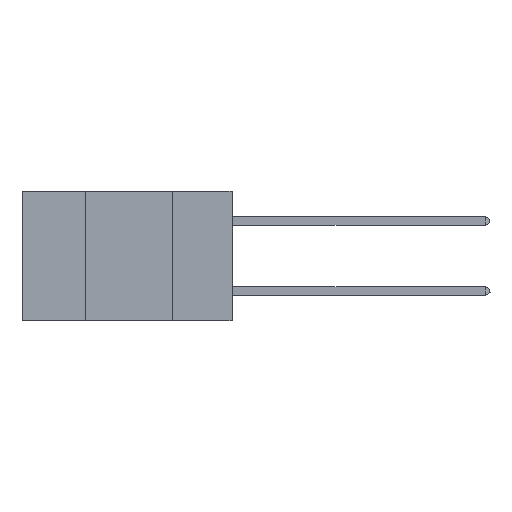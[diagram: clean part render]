
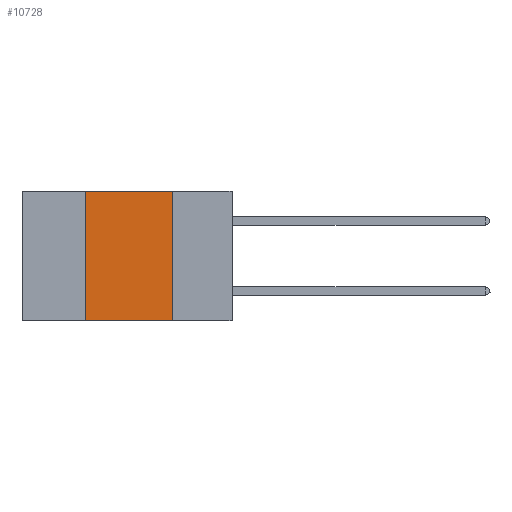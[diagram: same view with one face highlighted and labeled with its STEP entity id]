
A CAD part, left-side view. The second image highlights one B-rep face of the part: STEP entity #10728.
In plain terms, the highlighted planar face has unit normal (-1, 0, 0).
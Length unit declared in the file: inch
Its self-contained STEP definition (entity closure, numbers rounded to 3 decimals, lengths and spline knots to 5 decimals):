
#329 = CARTESIAN_POINT ( 'NONE',  ( 0., 0.17, -0.37 ) ) ;
#534 = LINE ( 'NONE', #3934, #16566 ) ;
#1298 = DIRECTION ( 'NONE',  ( 0., 0., -1. ) ) ;
#1723 = VECTOR ( 'NONE', #1298, 39.37008 ) ;
#2569 = VERTEX_POINT ( 'NONE', #2976 ) ;
#2976 = CARTESIAN_POINT ( 'NONE',  ( 0., 0.42, -0.37 ) ) ;
#3852 = CARTESIAN_POINT ( 'NONE',  ( 0., 0.42, 0. ) ) ;
#3934 = CARTESIAN_POINT ( 'NONE',  ( 0., 0.42, 0. ) ) ;
#4519 = ORIENTED_EDGE ( 'NONE', *, *, #20115, .T. ) ;
#4576 = CARTESIAN_POINT ( 'NONE',  ( 0., 0.17, 0. ) ) ;
#6358 = EDGE_CURVE ( 'NONE', #2569, #7148, #534, .T. ) ;
#6705 = DIRECTION ( 'NONE',  ( 1., 0., 0. ) ) ;
#7148 = VERTEX_POINT ( 'NONE', #3852 ) ;
#8247 = FACE_OUTER_BOUND ( 'NONE', #8736, .T. ) ;
#8339 = CARTESIAN_POINT ( 'NONE',  ( 0., 0.6, 0. ) ) ;
#8736 = EDGE_LOOP ( 'NONE', ( #20634, #13069, #10644, #4519 ) ) ;
#8959 = DIRECTION ( 'NONE',  ( 0., -1., 0. ) ) ;
#9198 = EDGE_CURVE ( 'NONE', #14615, #19133, #13212, .T. ) ;
#9330 = DIRECTION ( 'NONE',  ( 0., -1., 0. ) ) ;
#10610 = DIRECTION ( 'NONE',  ( 0., 0., 1. ) ) ;
#10644 = ORIENTED_EDGE ( 'NONE', *, *, #6358, .F. ) ;
#10728 = ADVANCED_FACE ( 'NONE', ( #8247 ), #11731, .F. ) ;
#10904 = AXIS2_PLACEMENT_3D ( 'NONE', #8339, #6705, #11299 ) ;
#10975 = CARTESIAN_POINT ( 'NONE',  ( 0., 0.6, -0.37 ) ) ;
#11299 = DIRECTION ( 'NONE',  ( 0., 0., -1. ) ) ;
#11504 = EDGE_CURVE ( 'NONE', #7148, #14615, #15724, .T. ) ;
#11731 = PLANE ( 'NONE',  #10904 ) ;
#11969 = VECTOR ( 'NONE', #9330, 39.37008 ) ;
#12699 = CARTESIAN_POINT ( 'NONE',  ( 0., 0.17, 0. ) ) ;
#13069 = ORIENTED_EDGE ( 'NONE', *, *, #11504, .F. ) ;
#13212 = LINE ( 'NONE', #4576, #1723 ) ;
#14615 = VERTEX_POINT ( 'NONE', #12699 ) ;
#15724 = LINE ( 'NONE', #20989, #18235 ) ;
#16222 = LINE ( 'NONE', #10975, #11969 ) ;
#16566 = VECTOR ( 'NONE', #10610, 39.37008 ) ;
#18235 = VECTOR ( 'NONE', #8959, 39.37008 ) ;
#19133 = VERTEX_POINT ( 'NONE', #329 ) ;
#20115 = EDGE_CURVE ( 'NONE', #2569, #19133, #16222, .T. ) ;
#20634 = ORIENTED_EDGE ( 'NONE', *, *, #9198, .F. ) ;
#20989 = CARTESIAN_POINT ( 'NONE',  ( 0., 0.6, 0. ) ) ;
